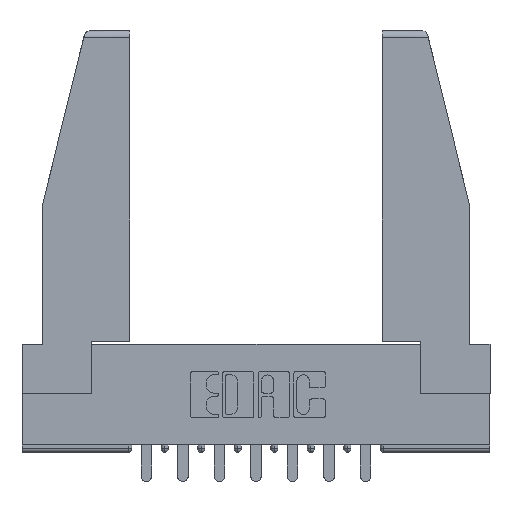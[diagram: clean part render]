
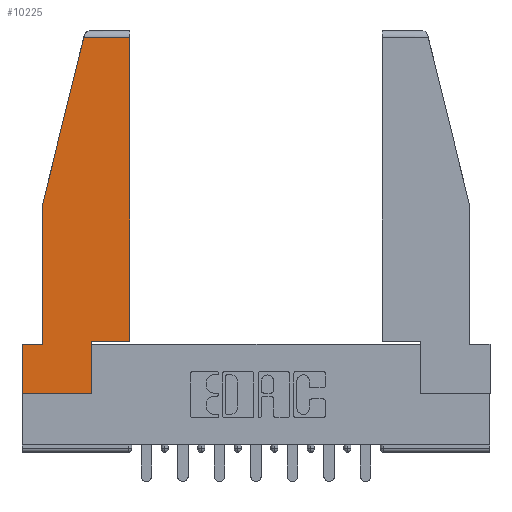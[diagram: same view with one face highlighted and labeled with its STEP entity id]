
A CAD part, top view. The second image highlights one B-rep face of the part: STEP entity #10225.
In plain terms, the highlighted planar face has unit normal (0, 0, 1).
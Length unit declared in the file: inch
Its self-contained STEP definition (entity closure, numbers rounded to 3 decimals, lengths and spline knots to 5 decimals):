
#8 = VERTEX_POINT ( 'NONE', #13003 ) ;
#174 = LINE ( 'NONE', #5593, #5814 ) ;
#247 = EDGE_CURVE ( 'NONE', #6908, #7292, #11047, .T. ) ;
#660 = CARTESIAN_POINT ( 'NONE',  ( 0.086, 0.8, 0. ) ) ;
#916 = DIRECTION ( 'NONE',  ( -0.239, -0.971, 0. ) ) ;
#920 = ORIENTED_EDGE ( 'NONE', *, *, #5818, .T. ) ;
#2029 = VERTEX_POINT ( 'NONE', #10159 ) ;
#2465 = DIRECTION ( 'NONE',  ( 0., 1., 0. ) ) ;
#2943 = VERTEX_POINT ( 'NONE', #10871 ) ;
#3090 = EDGE_CURVE ( 'NONE', #8362, #6766, #13925, .T. ) ;
#3381 = VECTOR ( 'NONE', #12499, 39.37008 ) ;
#3474 = CARTESIAN_POINT ( 'NONE',  ( 0.297, 0., 0. ) ) ;
#3636 = EDGE_CURVE ( 'NONE', #7483, #2029, #13210, .T. ) ;
#3747 = DIRECTION ( 'NONE',  ( 0., -1., 0. ) ) ;
#3810 = CARTESIAN_POINT ( 'NONE',  ( 0.461, 0.223, 0. ) ) ;
#3906 = CARTESIAN_POINT ( 'NONE',  ( 0., 0., 0. ) ) ;
#3937 = VECTOR ( 'NONE', #9842, 39.37008 ) ;
#4862 = CARTESIAN_POINT ( 'NONE',  ( 0., 1.52, 0. ) ) ;
#4908 = ORIENTED_EDGE ( 'NONE', *, *, #3090, .T. ) ;
#5460 = LINE ( 'NONE', #4862, #3381 ) ;
#5528 = CARTESIAN_POINT ( 'NONE',  ( 0., 0.21, 0. ) ) ;
#5587 = CARTESIAN_POINT ( 'NONE',  ( 0.2636, 1.52, 0. ) ) ;
#5593 = CARTESIAN_POINT ( 'NONE',  ( 0., 0.21, 0. ) ) ;
#5756 = CARTESIAN_POINT ( 'NONE',  ( 0.461, 0.223, 0. ) ) ;
#5812 = VECTOR ( 'NONE', #6143, 39.37008 ) ;
#5814 = VECTOR ( 'NONE', #3747, 39.37008 ) ;
#5818 = EDGE_CURVE ( 'NONE', #7292, #2943, #13946, .T. ) ;
#6143 = DIRECTION ( 'NONE',  ( 0., -1., 0. ) ) ;
#6261 = ORIENTED_EDGE ( 'NONE', *, *, #13568, .T. ) ;
#6299 = CARTESIAN_POINT ( 'NONE',  ( 0.297, 0., 0. ) ) ;
#6313 = LINE ( 'NONE', #9481, #14013 ) ;
#6687 = ORIENTED_EDGE ( 'NONE', *, *, #247, .T. ) ;
#6766 = VERTEX_POINT ( 'NONE', #7066 ) ;
#6908 = VERTEX_POINT ( 'NONE', #9188 ) ;
#7066 = CARTESIAN_POINT ( 'NONE',  ( 0., 0.21, 0. ) ) ;
#7138 = VECTOR ( 'NONE', #9530, 39.37008 ) ;
#7163 = ORIENTED_EDGE ( 'NONE', *, *, #3636, .T. ) ;
#7292 = VERTEX_POINT ( 'NONE', #6299 ) ;
#7343 = DIRECTION ( 'NONE',  ( 0., 0., 1. ) ) ;
#7388 = VECTOR ( 'NONE', #13765, 39.37008 ) ;
#7483 = VERTEX_POINT ( 'NONE', #5756 ) ;
#8027 = LINE ( 'NONE', #660, #5812 ) ;
#8362 = VERTEX_POINT ( 'NONE', #9429 ) ;
#8736 = EDGE_CURVE ( 'NONE', #2029, #10360, #5460, .T. ) ;
#9188 = CARTESIAN_POINT ( 'NONE',  ( 0., 0., 0. ) ) ;
#9208 = EDGE_CURVE ( 'NONE', #10360, #8, #6313, .T. ) ;
#9429 = CARTESIAN_POINT ( 'NONE',  ( 0.086, 0.21, 0. ) ) ;
#9481 = CARTESIAN_POINT ( 'NONE',  ( 0.271, 1.55, 0. ) ) ;
#9491 = CARTESIAN_POINT ( 'NONE',  ( 0., 0., 0. ) ) ;
#9518 = DIRECTION ( 'NONE',  ( 1., 0., 0. ) ) ;
#9530 = DIRECTION ( 'NONE',  ( 1., 0., 0. ) ) ;
#9842 = DIRECTION ( 'NONE',  ( -1., 0., 0. ) ) ;
#10159 = CARTESIAN_POINT ( 'NONE',  ( 0.461, 1.52, 0. ) ) ;
#10225 = ADVANCED_FACE ( 'NONE', ( #10870 ), #11482, .T. ) ;
#10297 = EDGE_LOOP ( 'NONE', ( #7163, #12353, #11433, #10390, #4908, #6261, #6687, #920, #12276 ) ) ;
#10360 = VERTEX_POINT ( 'NONE', #5587 ) ;
#10390 = ORIENTED_EDGE ( 'NONE', *, *, #12840, .T. ) ;
#10433 = CARTESIAN_POINT ( 'NONE',  ( 0.297, 0.223, 0. ) ) ;
#10839 = EDGE_CURVE ( 'NONE', #2943, #7483, #12553, .T. ) ;
#10870 = FACE_OUTER_BOUND ( 'NONE', #10297, .T. ) ;
#10871 = CARTESIAN_POINT ( 'NONE',  ( 0.297, 0.223, 0. ) ) ;
#11047 = LINE ( 'NONE', #9491, #7138 ) ;
#11433 = ORIENTED_EDGE ( 'NONE', *, *, #9208, .T. ) ;
#11482 = PLANE ( 'NONE',  #11786 ) ;
#11525 = DIRECTION ( 'NONE',  ( 1., 0., 0. ) ) ;
#11786 = AXIS2_PLACEMENT_3D ( 'NONE', #3906, #7343, #9518 ) ;
#12276 = ORIENTED_EDGE ( 'NONE', *, *, #10839, .T. ) ;
#12353 = ORIENTED_EDGE ( 'NONE', *, *, #8736, .T. ) ;
#12499 = DIRECTION ( 'NONE',  ( -1., 0., 0. ) ) ;
#12553 = LINE ( 'NONE', #10433, #14142 ) ;
#12703 = VECTOR ( 'NONE', #2465, 39.37008 ) ;
#12840 = EDGE_CURVE ( 'NONE', #8, #8362, #8027, .T. ) ;
#13003 = CARTESIAN_POINT ( 'NONE',  ( 0.086, 0.8, 0. ) ) ;
#13210 = LINE ( 'NONE', #3810, #7388 ) ;
#13568 = EDGE_CURVE ( 'NONE', #6766, #6908, #174, .T. ) ;
#13765 = DIRECTION ( 'NONE',  ( 0., 1., 0. ) ) ;
#13925 = LINE ( 'NONE', #5528, #3937 ) ;
#13946 = LINE ( 'NONE', #3474, #12703 ) ;
#14013 = VECTOR ( 'NONE', #916, 39.37008 ) ;
#14142 = VECTOR ( 'NONE', #11525, 39.37008 ) ;
